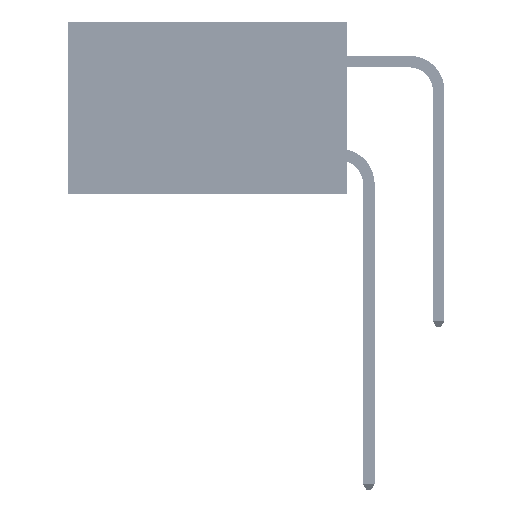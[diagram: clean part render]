
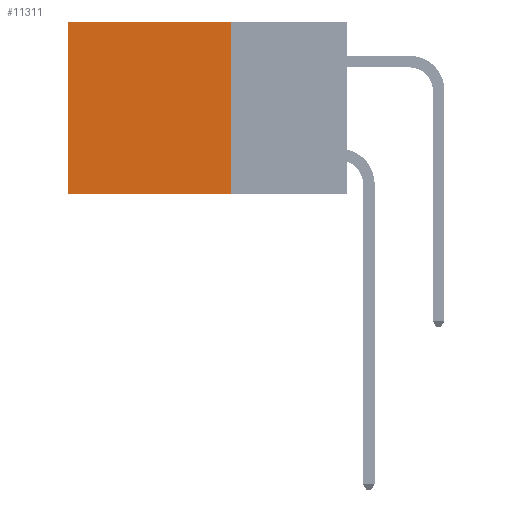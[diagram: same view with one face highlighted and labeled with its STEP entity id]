
A CAD part, left-side view. The second image highlights one B-rep face of the part: STEP entity #11311.
In plain terms, the highlighted planar face has unit normal (-1, 0, 0).
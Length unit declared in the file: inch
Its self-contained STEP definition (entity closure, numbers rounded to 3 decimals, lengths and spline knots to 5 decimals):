
#3856 = CARTESIAN_POINT ( 'NONE',  ( 0.2875, 0.25, -0.37 ) ) ;
#4207 = DIRECTION ( 'NONE',  ( 0., 0., -1. ) ) ;
#4373 = VERTEX_POINT ( 'NONE', #17389 ) ;
#4939 = ORIENTED_EDGE ( 'NONE', *, *, #40900, .T. ) ;
#5165 = LINE ( 'NONE', #25983, #41549 ) ;
#6189 = VECTOR ( 'NONE', #19805, 39.37008 ) ;
#10524 = DIRECTION ( 'NONE',  ( 0., 1., 0. ) ) ;
#11311 = ADVANCED_FACE ( 'NONE', ( #22816 ), #12218, .F. ) ;
#12218 = PLANE ( 'NONE',  #39332 ) ;
#12376 = DIRECTION ( 'NONE',  ( 1., 0., 0. ) ) ;
#13480 = ORIENTED_EDGE ( 'NONE', *, *, #42836, .F. ) ;
#16259 = VERTEX_POINT ( 'NONE', #34379 ) ;
#17389 = CARTESIAN_POINT ( 'NONE',  ( 0.2875, 0.6, -0.37 ) ) ;
#19805 = DIRECTION ( 'NONE',  ( 0., 1., 0. ) ) ;
#20183 = LINE ( 'NONE', #32155, #41236 ) ;
#20276 = CARTESIAN_POINT ( 'NONE',  ( 0.2875, 0.25, -0.37 ) ) ;
#21865 = VECTOR ( 'NONE', #38427, 39.37008 ) ;
#22042 = LINE ( 'NONE', #20276, #6189 ) ;
#22816 = FACE_OUTER_BOUND ( 'NONE', #25580, .T. ) ;
#23179 = DIRECTION ( 'NONE',  ( 0., 0., -1. ) ) ;
#23181 = EDGE_CURVE ( 'NONE', #26819, #4373, #22042, .T. ) ;
#25580 = EDGE_LOOP ( 'NONE', ( #46293, #35199, #13480, #4939 ) ) ;
#25983 = CARTESIAN_POINT ( 'NONE',  ( 0.2875, 0.6, 0. ) ) ;
#26819 = VERTEX_POINT ( 'NONE', #3856 ) ;
#31166 = EDGE_CURVE ( 'NONE', #35838, #4373, #5165, .T. ) ;
#32155 = CARTESIAN_POINT ( 'NONE',  ( 0.2875, 0.25, 0. ) ) ;
#33074 = CARTESIAN_POINT ( 'NONE',  ( 0.2875, 0.6, 0. ) ) ;
#34379 = CARTESIAN_POINT ( 'NONE',  ( 0.2875, 0.25, 0. ) ) ;
#35199 = ORIENTED_EDGE ( 'NONE', *, *, #23181, .F. ) ;
#35838 = VERTEX_POINT ( 'NONE', #33074 ) ;
#38427 = DIRECTION ( 'NONE',  ( 0., 0., -1. ) ) ;
#39332 = AXIS2_PLACEMENT_3D ( 'NONE', #41321, #12376, #23179 ) ;
#40152 = LINE ( 'NONE', #42243, #21865 ) ;
#40900 = EDGE_CURVE ( 'NONE', #16259, #35838, #20183, .T. ) ;
#41236 = VECTOR ( 'NONE', #10524, 39.37008 ) ;
#41321 = CARTESIAN_POINT ( 'NONE',  ( 0.2875, 0.25, 0. ) ) ;
#41549 = VECTOR ( 'NONE', #4207, 39.37008 ) ;
#42243 = CARTESIAN_POINT ( 'NONE',  ( 0.2875, 0.25, 0. ) ) ;
#42836 = EDGE_CURVE ( 'NONE', #16259, #26819, #40152, .T. ) ;
#46293 = ORIENTED_EDGE ( 'NONE', *, *, #31166, .T. ) ;
